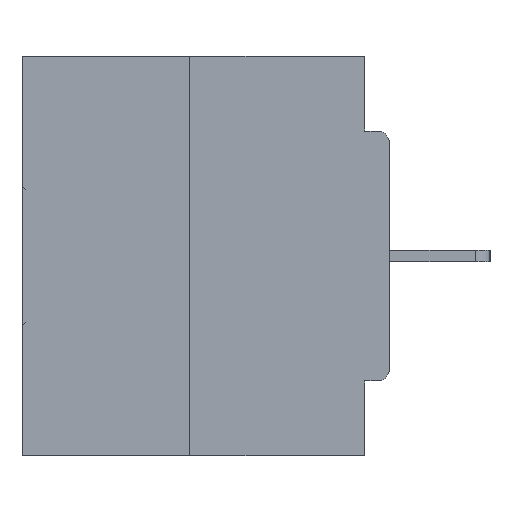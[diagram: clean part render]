
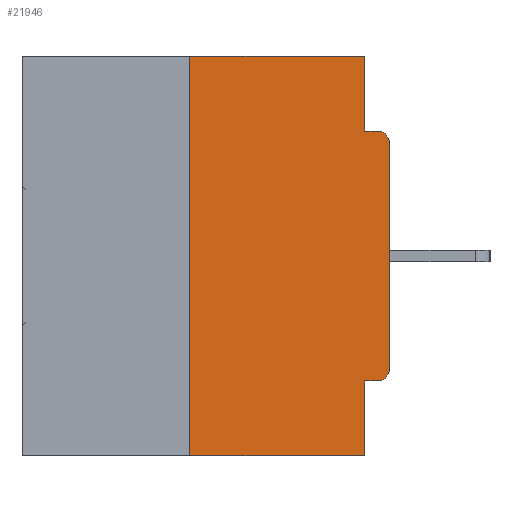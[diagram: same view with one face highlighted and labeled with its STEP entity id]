
A CAD part, left-side view. The second image highlights one B-rep face of the part: STEP entity #21946.
In plain terms, the highlighted planar face has unit normal (-1, 0, 0).
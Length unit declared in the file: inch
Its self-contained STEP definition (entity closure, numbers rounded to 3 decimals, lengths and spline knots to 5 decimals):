
#1142 = DIRECTION ( 'NONE',  ( 0., 0., 1. ) ) ;
#1183 = CARTESIAN_POINT ( 'NONE',  ( 0., 0.031, -0.5 ) ) ;
#1585 = VECTOR ( 'NONE', #10379, 39.37008 ) ;
#2768 = EDGE_CURVE ( 'NONE', #12576, #30592, #27061, .T. ) ;
#2984 = VERTEX_POINT ( 'NONE', #3148 ) ;
#3075 = CARTESIAN_POINT ( 'NONE',  ( 0., 0.25, 0. ) ) ;
#3148 = CARTESIAN_POINT ( 'NONE',  ( 0., 0., -0.3915 ) ) ;
#3508 = CARTESIAN_POINT ( 'NONE',  ( 0., 0., -0.1085 ) ) ;
#3735 = AXIS2_PLACEMENT_3D ( 'NONE', #4580, #21852, #18856 ) ;
#3899 = LINE ( 'NONE', #18761, #33382 ) ;
#4207 = PLANE ( 'NONE',  #3735 ) ;
#4365 = DIRECTION ( 'NONE',  ( 0., -1., 0. ) ) ;
#4580 = CARTESIAN_POINT ( 'NONE',  ( 0., 0.46, 0. ) ) ;
#4714 = VERTEX_POINT ( 'NONE', #1183 ) ;
#5477 = CARTESIAN_POINT ( 'NONE',  ( 0., 0.25, 0. ) ) ;
#6256 = DIRECTION ( 'NONE',  ( 0., 1., 0. ) ) ;
#6981 = CARTESIAN_POINT ( 'NONE',  ( 0., 0.031, -0.0935 ) ) ;
#7147 = EDGE_CURVE ( 'NONE', #21416, #20788, #33255, .T. ) ;
#9096 = DIRECTION ( 'NONE',  ( 0., 0., -1. ) ) ;
#9586 = CARTESIAN_POINT ( 'NONE',  ( 0., 0., -0.4065 ) ) ;
#10215 = CARTESIAN_POINT ( 'NONE',  ( 0., 0.46, 0. ) ) ;
#10262 = CARTESIAN_POINT ( 'NONE',  ( 0., 0.031, 0. ) ) ;
#10379 = DIRECTION ( 'NONE',  ( 0., 0., -1. ) ) ;
#10686 = EDGE_CURVE ( 'NONE', #14508, #26409, #21676, .T. ) ;
#11116 = CARTESIAN_POINT ( 'NONE',  ( 0., 0.031, 0. ) ) ;
#12068 = ORIENTED_EDGE ( 'NONE', *, *, #20715, .F. ) ;
#12183 = ORIENTED_EDGE ( 'NONE', *, *, #35132, .F. ) ;
#12325 = VERTEX_POINT ( 'NONE', #22465 ) ;
#12337 = EDGE_CURVE ( 'NONE', #20788, #4714, #27329, .T. ) ;
#12450 = DIRECTION ( 'NONE',  ( 0., -1., 0. ) ) ;
#12576 = VERTEX_POINT ( 'NONE', #11116 ) ;
#13174 = ORIENTED_EDGE ( 'NONE', *, *, #29152, .T. ) ;
#13202 = VECTOR ( 'NONE', #1142, 39.37008 ) ;
#13875 = DIRECTION ( 'NONE',  ( 0., 0., 1. ) ) ;
#14365 = VECTOR ( 'NONE', #13875, 39.37008 ) ;
#14508 = VERTEX_POINT ( 'NONE', #25947 ) ;
#14767 = CIRCLE ( 'NONE', #35439, 0.015 ) ;
#15926 = ORIENTED_EDGE ( 'NONE', *, *, #7147, .F. ) ;
#16088 = ORIENTED_EDGE ( 'NONE', *, *, #2768, .F. ) ;
#16109 = EDGE_CURVE ( 'NONE', #14508, #4714, #16686, .T. ) ;
#16686 = LINE ( 'NONE', #20800, #23363 ) ;
#16872 = ORIENTED_EDGE ( 'NONE', *, *, #16109, .T. ) ;
#17660 = ORIENTED_EDGE ( 'NONE', *, *, #10686, .F. ) ;
#17681 = CARTESIAN_POINT ( 'NONE',  ( 0., 0.015, -0.1085 ) ) ;
#18761 = CARTESIAN_POINT ( 'NONE',  ( 0., 0., -0.0935 ) ) ;
#18817 = ORIENTED_EDGE ( 'NONE', *, *, #27425, .T. ) ;
#18856 = DIRECTION ( 'NONE',  ( 0., 0., -1. ) ) ;
#20358 = AXIS2_PLACEMENT_3D ( 'NONE', #17681, #31843, #25890 ) ;
#20715 = EDGE_CURVE ( 'NONE', #30592, #12325, #3899, .T. ) ;
#20764 = CARTESIAN_POINT ( 'NONE',  ( 0., 0.015, -0.3915 ) ) ;
#20788 = VERTEX_POINT ( 'NONE', #27497 ) ;
#20800 = CARTESIAN_POINT ( 'NONE',  ( 0., 0.46, -0.5 ) ) ;
#21416 = VERTEX_POINT ( 'NONE', #32086 ) ;
#21676 = LINE ( 'NONE', #3075, #13202 ) ;
#21852 = DIRECTION ( 'NONE',  ( 1., 0., 0. ) ) ;
#21946 = ADVANCED_FACE ( 'NONE', ( #36837 ), #4207, .F. ) ;
#22465 = CARTESIAN_POINT ( 'NONE',  ( 0., 0.015, -0.0935 ) ) ;
#22549 = ORIENTED_EDGE ( 'NONE', *, *, #27897, .T. ) ;
#23363 = VECTOR ( 'NONE', #12450, 39.37008 ) ;
#23564 = CIRCLE ( 'NONE', #20358, 0.015 ) ;
#24505 = LINE ( 'NONE', #10215, #29911 ) ;
#24666 = VECTOR ( 'NONE', #33657, 39.37008 ) ;
#24989 = CARTESIAN_POINT ( 'NONE',  ( 0., 0.031, -0.5 ) ) ;
#25890 = DIRECTION ( 'NONE',  ( 0., 0., -1. ) ) ;
#25947 = CARTESIAN_POINT ( 'NONE',  ( 0., 0.25, -0.5 ) ) ;
#26409 = VERTEX_POINT ( 'NONE', #5477 ) ;
#26863 = LINE ( 'NONE', #36462, #14365 ) ;
#26888 = ORIENTED_EDGE ( 'NONE', *, *, #12337, .F. ) ;
#27061 = LINE ( 'NONE', #10262, #1585 ) ;
#27329 = LINE ( 'NONE', #24989, #24666 ) ;
#27425 = EDGE_CURVE ( 'NONE', #2984, #31165, #26863, .T. ) ;
#27497 = CARTESIAN_POINT ( 'NONE',  ( 0., 0.031, -0.4065 ) ) ;
#27897 = EDGE_CURVE ( 'NONE', #21416, #2984, #14767, .T. ) ;
#28272 = VECTOR ( 'NONE', #6256, 39.37008 ) ;
#28934 = EDGE_LOOP ( 'NONE', ( #12183, #17660, #16872, #26888, #15926, #22549, #18817, #13174, #12068, #16088 ) ) ;
#29152 = EDGE_CURVE ( 'NONE', #31165, #12325, #23564, .T. ) ;
#29911 = VECTOR ( 'NONE', #4365, 39.37008 ) ;
#30592 = VERTEX_POINT ( 'NONE', #6981 ) ;
#31165 = VERTEX_POINT ( 'NONE', #3508 ) ;
#31843 = DIRECTION ( 'NONE',  ( -1., 0., 0. ) ) ;
#32086 = CARTESIAN_POINT ( 'NONE',  ( 0., 0.015, -0.4065 ) ) ;
#33255 = LINE ( 'NONE', #9586, #28272 ) ;
#33382 = VECTOR ( 'NONE', #36059, 39.37008 ) ;
#33657 = DIRECTION ( 'NONE',  ( 0., 0., -1. ) ) ;
#34919 = DIRECTION ( 'NONE',  ( -1., 0., 0. ) ) ;
#35132 = EDGE_CURVE ( 'NONE', #26409, #12576, #24505, .T. ) ;
#35439 = AXIS2_PLACEMENT_3D ( 'NONE', #20764, #34919, #9096 ) ;
#36059 = DIRECTION ( 'NONE',  ( 0., -1., 0. ) ) ;
#36462 = CARTESIAN_POINT ( 'NONE',  ( 0., 0., 0. ) ) ;
#36837 = FACE_OUTER_BOUND ( 'NONE', #28934, .T. ) ;
